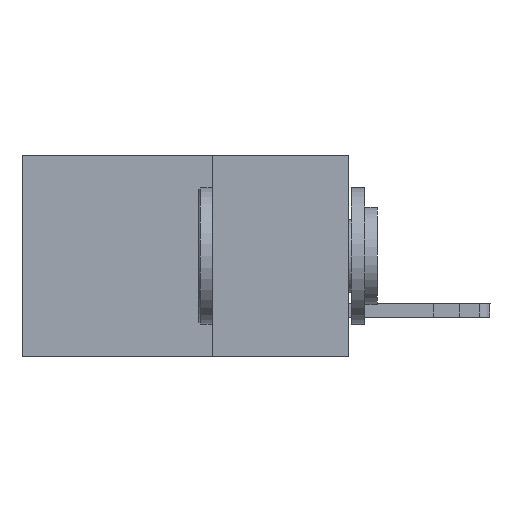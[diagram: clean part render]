
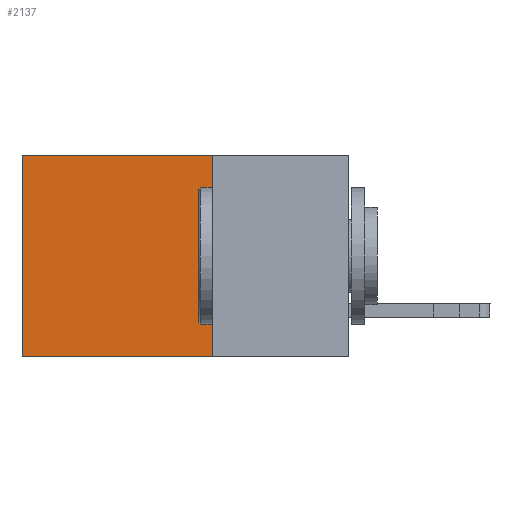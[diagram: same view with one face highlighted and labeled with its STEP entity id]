
A CAD part, left-side view. The second image highlights one B-rep face of the part: STEP entity #2137.
In plain terms, the highlighted planar face has unit normal (-1, 0, 0).
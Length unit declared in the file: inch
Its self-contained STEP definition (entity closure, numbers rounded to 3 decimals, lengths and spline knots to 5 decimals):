
#315 = VERTEX_POINT ( 'NONE', #18436 ) ;
#395 = VECTOR ( 'NONE', #14343, 39.37008 ) ;
#1009 = VERTEX_POINT ( 'NONE', #11575 ) ;
#1234 = DIRECTION ( 'NONE',  ( 1., 0., 0. ) ) ;
#2137 = ADVANCED_FACE ( 'NONE', ( #14106 ), #3718, .F. ) ;
#3718 = PLANE ( 'NONE',  #10459 ) ;
#4891 = CARTESIAN_POINT ( 'NONE',  ( 0.298, 0.25, 0. ) ) ;
#5054 = ORIENTED_EDGE ( 'NONE', *, *, #14040, .F. ) ;
#5349 = DIRECTION ( 'NONE',  ( 0., 0., -1. ) ) ;
#5394 = CARTESIAN_POINT ( 'NONE',  ( 0.298, 0.25, 0. ) ) ;
#5742 = ORIENTED_EDGE ( 'NONE', *, *, #12736, .T. ) ;
#6697 = LINE ( 'NONE', #12845, #10857 ) ;
#7491 = LINE ( 'NONE', #18546, #395 ) ;
#8697 = ORIENTED_EDGE ( 'NONE', *, *, #12852, .F. ) ;
#9013 = LINE ( 'NONE', #12292, #17407 ) ;
#9932 = CARTESIAN_POINT ( 'NONE',  ( 0.298, 0.6, 0. ) ) ;
#10116 = VECTOR ( 'NONE', #12630, 39.37008 ) ;
#10459 = AXIS2_PLACEMENT_3D ( 'NONE', #11043, #1234, #14356 ) ;
#10857 = VECTOR ( 'NONE', #15828, 39.37008 ) ;
#11043 = CARTESIAN_POINT ( 'NONE',  ( 0.298, 0.25, 0. ) ) ;
#11059 = EDGE_LOOP ( 'NONE', ( #5742, #8697, #5054, #14069 ) ) ;
#11491 = LINE ( 'NONE', #5394, #10116 ) ;
#11575 = CARTESIAN_POINT ( 'NONE',  ( 0.298, 0.25, -0.37 ) ) ;
#12292 = CARTESIAN_POINT ( 'NONE',  ( 0.298, 0.6, 0. ) ) ;
#12630 = DIRECTION ( 'NONE',  ( 0., 0., -1. ) ) ;
#12736 = EDGE_CURVE ( 'NONE', #13731, #315, #9013, .T. ) ;
#12845 = CARTESIAN_POINT ( 'NONE',  ( 0.298, 0.25, -0.37 ) ) ;
#12852 = EDGE_CURVE ( 'NONE', #1009, #315, #6697, .T. ) ;
#13731 = VERTEX_POINT ( 'NONE', #9932 ) ;
#14040 = EDGE_CURVE ( 'NONE', #18290, #1009, #11491, .T. ) ;
#14069 = ORIENTED_EDGE ( 'NONE', *, *, #16213, .T. ) ;
#14106 = FACE_OUTER_BOUND ( 'NONE', #11059, .T. ) ;
#14343 = DIRECTION ( 'NONE',  ( 0., 1., 0. ) ) ;
#14356 = DIRECTION ( 'NONE',  ( 0., 0., -1. ) ) ;
#15828 = DIRECTION ( 'NONE',  ( 0., 1., 0. ) ) ;
#16213 = EDGE_CURVE ( 'NONE', #18290, #13731, #7491, .T. ) ;
#17407 = VECTOR ( 'NONE', #5349, 39.37008 ) ;
#18290 = VERTEX_POINT ( 'NONE', #4891 ) ;
#18436 = CARTESIAN_POINT ( 'NONE',  ( 0.298, 0.6, -0.37 ) ) ;
#18546 = CARTESIAN_POINT ( 'NONE',  ( 0.298, 0.25, 0. ) ) ;
